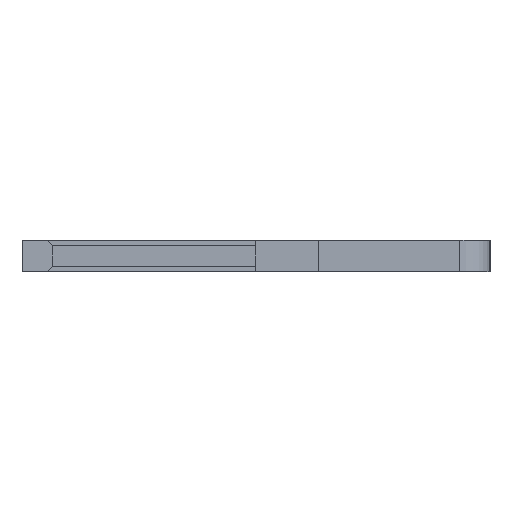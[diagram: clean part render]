
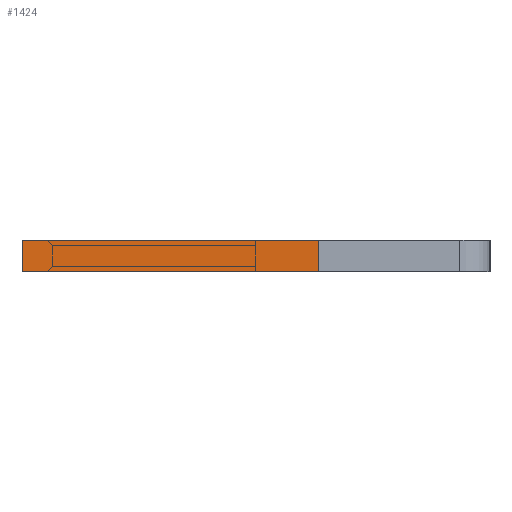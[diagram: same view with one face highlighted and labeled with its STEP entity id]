
A CAD part, left-side view. The second image highlights one B-rep face of the part: STEP entity #1424.
In plain terms, the highlighted face is planar.
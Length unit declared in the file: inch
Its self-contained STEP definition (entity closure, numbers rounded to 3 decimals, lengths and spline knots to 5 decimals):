
#190 = DIRECTION ( 'NONE',  ( -1., 0., 0. ) ) ;
#229 = DIRECTION ( 'NONE',  ( 1., 0., 0. ) ) ;
#400 = LINE ( 'NONE', #4090, #4076 ) ;
#452 = EDGE_LOOP ( 'NONE', ( #1226, #2028, #558, #3131 ) ) ;
#558 = ORIENTED_EDGE ( 'NONE', *, *, #3902, .F. ) ;
#606 = CARTESIAN_POINT ( 'NONE',  ( 0.01, 0.15, -0.04 ) ) ;
#690 = AXIS2_PLACEMENT_3D ( 'NONE', #3504, #3118, #229 ) ;
#694 = LINE ( 'NONE', #606, #3418 ) ;
#1101 = CARTESIAN_POINT ( 'NONE',  ( 0.01, -0.04, -0.04 ) ) ;
#1222 = EDGE_CURVE ( 'NONE', #3608, #1856, #400, .T. ) ;
#1226 = ORIENTED_EDGE ( 'NONE', *, *, #1222, .T. ) ;
#1314 = CARTESIAN_POINT ( 'NONE',  ( -0.01, 0.15, -0.04 ) ) ;
#1424 = ADVANCED_FACE ( 'NONE', ( #2691 ), #3057, .F. ) ;
#1693 = EDGE_CURVE ( 'NONE', #3407, #1856, #694, .T. ) ;
#1813 = CARTESIAN_POINT ( 'NONE',  ( 0.01, 0.15, -0.04 ) ) ;
#1833 = CARTESIAN_POINT ( 'NONE',  ( 0.01, 0.15, -0.04 ) ) ;
#1845 = LINE ( 'NONE', #4269, #2682 ) ;
#1856 = VERTEX_POINT ( 'NONE', #1314 ) ;
#1927 = CARTESIAN_POINT ( 'NONE',  ( -0.01, -0.04, -0.04 ) ) ;
#2028 = ORIENTED_EDGE ( 'NONE', *, *, #1693, .F. ) ;
#2109 = LINE ( 'NONE', #1833, #2939 ) ;
#2682 = VECTOR ( 'NONE', #190, 39.37008 ) ;
#2691 = FACE_OUTER_BOUND ( 'NONE', #452, .T. ) ;
#2939 = VECTOR ( 'NONE', #4340, 39.37008 ) ;
#2958 = EDGE_CURVE ( 'NONE', #4138, #3608, #1845, .T. ) ;
#3057 = PLANE ( 'NONE',  #690 ) ;
#3118 = DIRECTION ( 'NONE',  ( 0., 0., 1. ) ) ;
#3131 = ORIENTED_EDGE ( 'NONE', *, *, #2958, .T. ) ;
#3407 = VERTEX_POINT ( 'NONE', #1813 ) ;
#3418 = VECTOR ( 'NONE', #3794, 39.37008 ) ;
#3504 = CARTESIAN_POINT ( 'NONE',  ( 0.01, 0.15, -0.04 ) ) ;
#3608 = VERTEX_POINT ( 'NONE', #1927 ) ;
#3794 = DIRECTION ( 'NONE',  ( -1., 0., 0. ) ) ;
#3902 = EDGE_CURVE ( 'NONE', #4138, #3407, #2109, .T. ) ;
#4076 = VECTOR ( 'NONE', #4434, 39.37008 ) ;
#4090 = CARTESIAN_POINT ( 'NONE',  ( -0.01, 0.15, -0.04 ) ) ;
#4138 = VERTEX_POINT ( 'NONE', #1101 ) ;
#4269 = CARTESIAN_POINT ( 'NONE',  ( 0.01, -0.04, -0.04 ) ) ;
#4340 = DIRECTION ( 'NONE',  ( 0., 1., 0. ) ) ;
#4434 = DIRECTION ( 'NONE',  ( 0., 1., 0. ) ) ;
